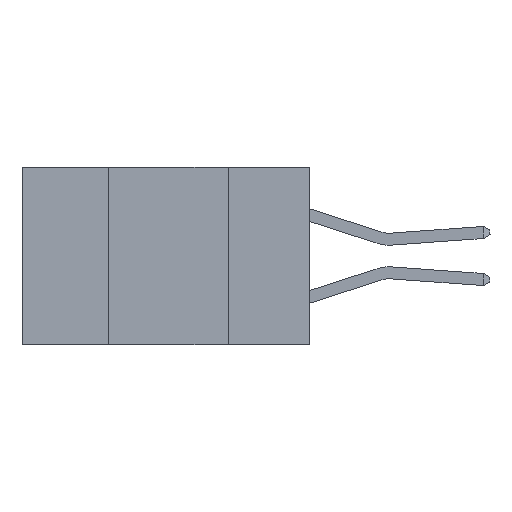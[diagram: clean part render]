
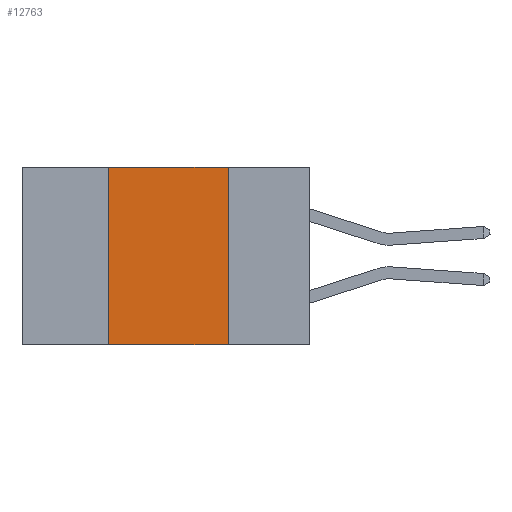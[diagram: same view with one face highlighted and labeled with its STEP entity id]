
A CAD part, left-side view. The second image highlights one B-rep face of the part: STEP entity #12763.
In plain terms, the highlighted planar face has unit normal (-1, 0, 0).
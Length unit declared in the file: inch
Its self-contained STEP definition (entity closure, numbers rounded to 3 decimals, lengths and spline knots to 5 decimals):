
#681 = CARTESIAN_POINT ( 'NONE',  ( 0., 0.17, 0. ) ) ;
#1021 = FACE_OUTER_BOUND ( 'NONE', #15354, .T. ) ;
#1058 = VECTOR ( 'NONE', #22727, 39.37008 ) ;
#1123 = LINE ( 'NONE', #15518, #1058 ) ;
#1168 = CARTESIAN_POINT ( 'NONE',  ( 0., 0.17, -0.37 ) ) ;
#1206 = VECTOR ( 'NONE', #1493, 39.37008 ) ;
#1493 = DIRECTION ( 'NONE',  ( 0., 0., -1. ) ) ;
#2323 = EDGE_CURVE ( 'NONE', #15238, #14755, #4907, .T. ) ;
#2947 = LINE ( 'NONE', #5073, #5882 ) ;
#3012 = VERTEX_POINT ( 'NONE', #11263 ) ;
#3822 = ORIENTED_EDGE ( 'NONE', *, *, #20543, .F. ) ;
#4905 = DIRECTION ( 'NONE',  ( 0., 0., -1. ) ) ;
#4907 = LINE ( 'NONE', #5023, #1206 ) ;
#5023 = CARTESIAN_POINT ( 'NONE',  ( 0., 0.17, -0.37 ) ) ;
#5073 = CARTESIAN_POINT ( 'NONE',  ( 0., 0.42, -0.37 ) ) ;
#5375 = CARTESIAN_POINT ( 'NONE',  ( 0., 0.6, -0.37 ) ) ;
#5882 = VECTOR ( 'NONE', #19592, 39.37008 ) ;
#5939 = ORIENTED_EDGE ( 'NONE', *, *, #9781, .T. ) ;
#6334 = VERTEX_POINT ( 'NONE', #13620 ) ;
#6347 = CARTESIAN_POINT ( 'NONE',  ( 0., 0.6, 0. ) ) ;
#6587 = DIRECTION ( 'NONE',  ( 1., 0., 0. ) ) ;
#8191 = ORIENTED_EDGE ( 'NONE', *, *, #2323, .F. ) ;
#8431 = AXIS2_PLACEMENT_3D ( 'NONE', #6347, #6587, #4905 ) ;
#9781 = EDGE_CURVE ( 'NONE', #3012, #14755, #21321, .T. ) ;
#10126 = EDGE_CURVE ( 'NONE', #3012, #6334, #2947, .T. ) ;
#11263 = CARTESIAN_POINT ( 'NONE',  ( 0., 0.42, -0.37 ) ) ;
#12763 = ADVANCED_FACE ( 'NONE', ( #1021 ), #13884, .F. ) ;
#13620 = CARTESIAN_POINT ( 'NONE',  ( 0., 0.42, 0. ) ) ;
#13884 = PLANE ( 'NONE',  #8431 ) ;
#14755 = VERTEX_POINT ( 'NONE', #1168 ) ;
#15238 = VERTEX_POINT ( 'NONE', #681 ) ;
#15354 = EDGE_LOOP ( 'NONE', ( #8191, #3822, #16609, #5939 ) ) ;
#15518 = CARTESIAN_POINT ( 'NONE',  ( 0., 0.6, 0. ) ) ;
#16609 = ORIENTED_EDGE ( 'NONE', *, *, #10126, .F. ) ;
#18710 = VECTOR ( 'NONE', #22976, 39.37008 ) ;
#19592 = DIRECTION ( 'NONE',  ( 0., 0., 1. ) ) ;
#20543 = EDGE_CURVE ( 'NONE', #6334, #15238, #1123, .T. ) ;
#21321 = LINE ( 'NONE', #5375, #18710 ) ;
#22727 = DIRECTION ( 'NONE',  ( 0., -1., 0. ) ) ;
#22976 = DIRECTION ( 'NONE',  ( 0., -1., 0. ) ) ;
